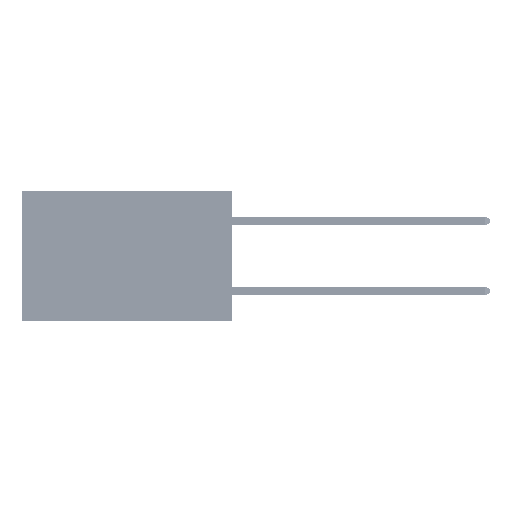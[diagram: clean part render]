
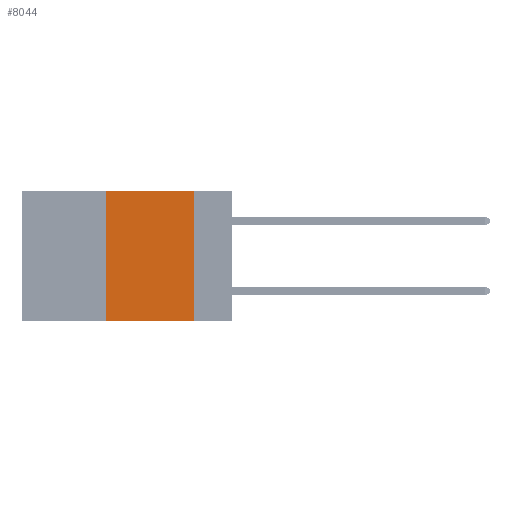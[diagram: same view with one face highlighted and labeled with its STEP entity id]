
A CAD part, left-side view. The second image highlights one B-rep face of the part: STEP entity #8044.
In plain terms, the highlighted planar face has unit normal (-1, 0, 0).
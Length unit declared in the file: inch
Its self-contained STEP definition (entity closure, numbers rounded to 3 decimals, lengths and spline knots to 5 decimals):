
#451 = LINE ( 'NONE', #26275, #37148 ) ;
#462 = ORIENTED_EDGE ( 'NONE', *, *, #7623, .T. ) ;
#844 = CARTESIAN_POINT ( 'NONE',  ( 0., 0.36, -0.37 ) ) ;
#1901 = ORIENTED_EDGE ( 'NONE', *, *, #17964, .F. ) ;
#2643 = LINE ( 'NONE', #13406, #25164 ) ;
#4230 = EDGE_LOOP ( 'NONE', ( #1901, #34314, #46800, #462 ) ) ;
#4478 = LINE ( 'NONE', #4953, #9016 ) ;
#4953 = CARTESIAN_POINT ( 'NONE',  ( 0., 0.6, 0. ) ) ;
#7623 = EDGE_CURVE ( 'NONE', #9614, #27355, #20286, .T. ) ;
#8044 = ADVANCED_FACE ( 'NONE', ( #38851 ), #20927, .F. ) ;
#9016 = VECTOR ( 'NONE', #11882, 39.37008 ) ;
#9614 = VERTEX_POINT ( 'NONE', #844 ) ;
#9704 = DIRECTION ( 'NONE',  ( 1., 0., 0. ) ) ;
#9753 = CARTESIAN_POINT ( 'NONE',  ( 0., 0.6, -0.37 ) ) ;
#11882 = DIRECTION ( 'NONE',  ( 0., -1., 0. ) ) ;
#12786 = EDGE_CURVE ( 'NONE', #9614, #33965, #451, .T. ) ;
#13406 = CARTESIAN_POINT ( 'NONE',  ( 0., 0.11, 0. ) ) ;
#17224 = DIRECTION ( 'NONE',  ( 0., 0., -1. ) ) ;
#17860 = VECTOR ( 'NONE', #38671, 39.37008 ) ;
#17964 = EDGE_CURVE ( 'NONE', #20940, #27355, #2643, .T. ) ;
#20286 = LINE ( 'NONE', #9753, #17860 ) ;
#20927 = PLANE ( 'NONE',  #43801 ) ;
#20940 = VERTEX_POINT ( 'NONE', #27770 ) ;
#21509 = DIRECTION ( 'NONE',  ( 0., 0., 1. ) ) ;
#25164 = VECTOR ( 'NONE', #17224, 39.37008 ) ;
#26275 = CARTESIAN_POINT ( 'NONE',  ( 0., 0.36, 0. ) ) ;
#27355 = VERTEX_POINT ( 'NONE', #44211 ) ;
#27770 = CARTESIAN_POINT ( 'NONE',  ( 0., 0.11, 0. ) ) ;
#31686 = CARTESIAN_POINT ( 'NONE',  ( 0., 0.36, 0. ) ) ;
#33965 = VERTEX_POINT ( 'NONE', #31686 ) ;
#34314 = ORIENTED_EDGE ( 'NONE', *, *, #37008, .F. ) ;
#35520 = DIRECTION ( 'NONE',  ( 0., 0., -1. ) ) ;
#37008 = EDGE_CURVE ( 'NONE', #33965, #20940, #4478, .T. ) ;
#37148 = VECTOR ( 'NONE', #21509, 39.37008 ) ;
#38671 = DIRECTION ( 'NONE',  ( 0., -1., 0. ) ) ;
#38851 = FACE_OUTER_BOUND ( 'NONE', #4230, .T. ) ;
#43801 = AXIS2_PLACEMENT_3D ( 'NONE', #45554, #9704, #35520 ) ;
#44211 = CARTESIAN_POINT ( 'NONE',  ( 0., 0.11, -0.37 ) ) ;
#45554 = CARTESIAN_POINT ( 'NONE',  ( 0., 0.6, 0. ) ) ;
#46800 = ORIENTED_EDGE ( 'NONE', *, *, #12786, .F. ) ;
